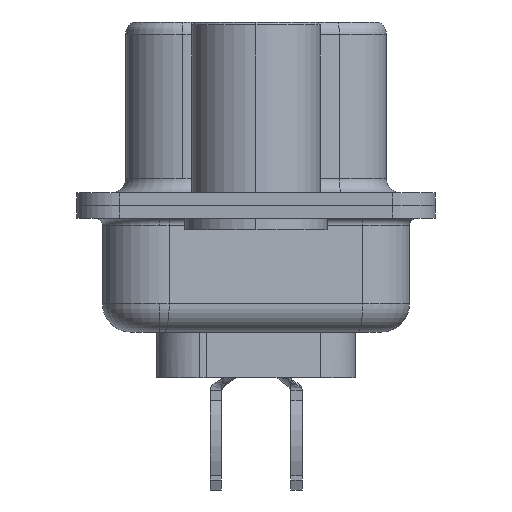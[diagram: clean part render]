
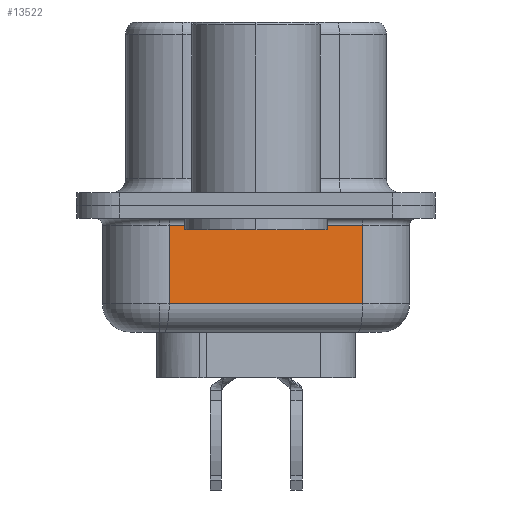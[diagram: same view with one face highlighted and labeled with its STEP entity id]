
A CAD part, left-side view. The second image highlights one B-rep face of the part: STEP entity #13522.
In plain terms, the highlighted planar face has unit normal (-0.985, -0.174, 0).
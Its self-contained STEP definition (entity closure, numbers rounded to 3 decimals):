
#67 = CARTESIAN_POINT ( 'NONE',  ( 2.875, 3.053, -3.45 ) ) ;
#184 = ORIENTED_EDGE ( 'NONE', *, *, #3535, .F. ) ;
#240 = LINE ( 'NONE', #67, #10633 ) ;
#920 = EDGE_CURVE ( 'NONE', #2088, #10962, #240, .T. ) ;
#2088 = VERTEX_POINT ( 'NONE', #2514 ) ;
#2364 = FACE_OUTER_BOUND ( 'NONE', #7246, .T. ) ;
#2514 = CARTESIAN_POINT ( 'NONE',  ( 2.875, 3.053, -3.45 ) ) ;
#3009 = VECTOR ( 'NONE', #9764, 1000. ) ;
#3535 = EDGE_CURVE ( 'NONE', #2088, #9102, #16906, .T. ) ;
#4375 = VECTOR ( 'NONE', #12064, 1000. ) ;
#4717 = DIRECTION ( 'NONE',  ( 0.985, 0.174, 0. ) ) ;
#4983 = DIRECTION ( 'NONE',  ( -0.174, 0.985, 0. ) ) ;
#5822 = ORIENTED_EDGE ( 'NONE', *, *, #920, .T. ) ;
#5895 = CARTESIAN_POINT ( 'NONE',  ( 2.875, 3.053, -0.7 ) ) ;
#5971 = DIRECTION ( 'NONE',  ( -0.174, 0.985, 0. ) ) ;
#7246 = EDGE_LOOP ( 'NONE', ( #184, #5822, #17473, #10308 ) ) ;
#7934 = CARTESIAN_POINT ( 'NONE',  ( 4.074, -3.747, -4.45 ) ) ;
#8216 = DIRECTION ( 'NONE',  ( 0.174, -0.985, 0. ) ) ;
#8251 = CARTESIAN_POINT ( 'NONE',  ( 2.875, 3.053, -4.45 ) ) ;
#9102 = VERTEX_POINT ( 'NONE', #10695 ) ;
#9764 = DIRECTION ( 'NONE',  ( 0., 0., 1. ) ) ;
#10308 = ORIENTED_EDGE ( 'NONE', *, *, #17323, .T. ) ;
#10526 = PLANE ( 'NONE',  #16405 ) ;
#10633 = VECTOR ( 'NONE', #8216, 1000. ) ;
#10695 = CARTESIAN_POINT ( 'NONE',  ( 2.875, 3.053, -0.7 ) ) ;
#10962 = VERTEX_POINT ( 'NONE', #13123 ) ;
#11785 = CARTESIAN_POINT ( 'NONE',  ( 2.875, 3.053, -4.45 ) ) ;
#12064 = DIRECTION ( 'NONE',  ( 0., 0., 1. ) ) ;
#12256 = VERTEX_POINT ( 'NONE', #12983 ) ;
#12983 = CARTESIAN_POINT ( 'NONE',  ( 4.074, -3.747, -0.7 ) ) ;
#13123 = CARTESIAN_POINT ( 'NONE',  ( 4.074, -3.747, -3.45 ) ) ;
#13522 = ADVANCED_FACE ( 'NONE', ( #2364 ), #10526, .F. ) ;
#15287 = EDGE_CURVE ( 'NONE', #10962, #12256, #16159, .T. ) ;
#15328 = VECTOR ( 'NONE', #5971, 1000. ) ;
#15541 = LINE ( 'NONE', #5895, #15328 ) ;
#16159 = LINE ( 'NONE', #7934, #4375 ) ;
#16405 = AXIS2_PLACEMENT_3D ( 'NONE', #11785, #4717, #4983 ) ;
#16906 = LINE ( 'NONE', #8251, #3009 ) ;
#17323 = EDGE_CURVE ( 'NONE', #12256, #9102, #15541, .T. ) ;
#17473 = ORIENTED_EDGE ( 'NONE', *, *, #15287, .T. ) ;
